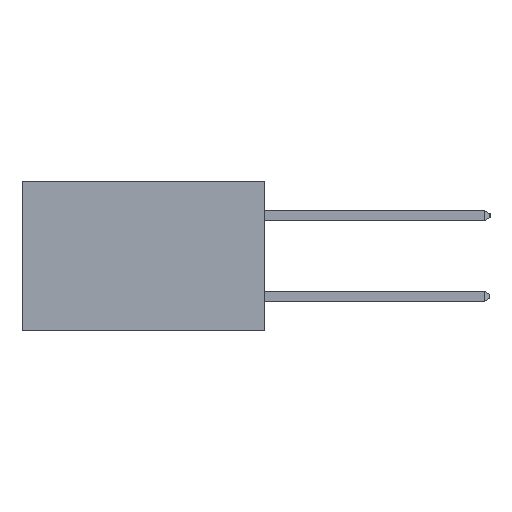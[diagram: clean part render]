
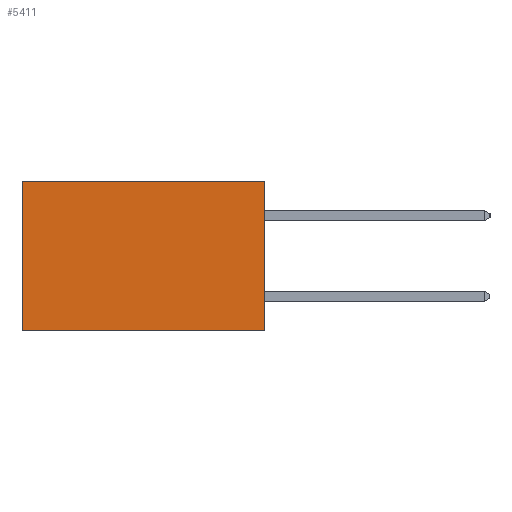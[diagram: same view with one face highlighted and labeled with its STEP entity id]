
A CAD part, left-side view. The second image highlights one B-rep face of the part: STEP entity #5411.
In plain terms, the highlighted planar face has unit normal (-1, 0, 0).
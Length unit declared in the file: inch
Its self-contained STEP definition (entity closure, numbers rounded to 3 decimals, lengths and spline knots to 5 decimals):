
#202 = VECTOR ( 'NONE', #15864, 39.37008 ) ;
#909 = EDGE_CURVE ( 'NONE', #8495, #8430, #10309, .T. ) ;
#1113 = DIRECTION ( 'NONE',  ( 1., 0., 0. ) ) ;
#1303 = CARTESIAN_POINT ( 'NONE',  ( 0.2615, 0., -0.37 ) ) ;
#1357 = LINE ( 'NONE', #3904, #6121 ) ;
#1825 = LINE ( 'NONE', #8540, #7843 ) ;
#2443 = DIRECTION ( 'NONE',  ( 0., 0., -1. ) ) ;
#2485 = ORIENTED_EDGE ( 'NONE', *, *, #9962, .T. ) ;
#3887 = AXIS2_PLACEMENT_3D ( 'NONE', #6572, #1113, #17454 ) ;
#3904 = CARTESIAN_POINT ( 'NONE',  ( 0.2615, 0., 0. ) ) ;
#4393 = EDGE_CURVE ( 'NONE', #8430, #11724, #10046, .T. ) ;
#4702 = ORIENTED_EDGE ( 'NONE', *, *, #5030, .T. ) ;
#5030 = EDGE_CURVE ( 'NONE', #6061, #11724, #1825, .T. ) ;
#5411 = ADVANCED_FACE ( 'NONE', ( #8099 ), #13270, .F. ) ;
#6061 = VERTEX_POINT ( 'NONE', #8173 ) ;
#6121 = VECTOR ( 'NONE', #13860, 39.37008 ) ;
#6231 = CARTESIAN_POINT ( 'NONE',  ( 0.2615, 0., -0.37 ) ) ;
#6572 = CARTESIAN_POINT ( 'NONE',  ( 0.2615, 0., -0.37 ) ) ;
#6700 = VECTOR ( 'NONE', #2443, 39.37008 ) ;
#7843 = VECTOR ( 'NONE', #12641, 39.37008 ) ;
#8099 = FACE_OUTER_BOUND ( 'NONE', #14757, .T. ) ;
#8173 = CARTESIAN_POINT ( 'NONE',  ( 0.2615, 0.6, 0. ) ) ;
#8430 = VERTEX_POINT ( 'NONE', #1303 ) ;
#8495 = VERTEX_POINT ( 'NONE', #13818 ) ;
#8540 = CARTESIAN_POINT ( 'NONE',  ( 0.2615, 0.6, -0.37 ) ) ;
#9392 = ORIENTED_EDGE ( 'NONE', *, *, #909, .F. ) ;
#9962 = EDGE_CURVE ( 'NONE', #8495, #6061, #1357, .T. ) ;
#10046 = LINE ( 'NONE', #6231, #202 ) ;
#10309 = LINE ( 'NONE', #15767, #6700 ) ;
#10592 = CARTESIAN_POINT ( 'NONE',  ( 0.2615, 0.6, -0.37 ) ) ;
#11724 = VERTEX_POINT ( 'NONE', #10592 ) ;
#12641 = DIRECTION ( 'NONE',  ( 0., 0., -1. ) ) ;
#13270 = PLANE ( 'NONE',  #3887 ) ;
#13818 = CARTESIAN_POINT ( 'NONE',  ( 0.2615, 0., 0. ) ) ;
#13860 = DIRECTION ( 'NONE',  ( 0., 1., 0. ) ) ;
#14757 = EDGE_LOOP ( 'NONE', ( #4702, #15365, #9392, #2485 ) ) ;
#15365 = ORIENTED_EDGE ( 'NONE', *, *, #4393, .F. ) ;
#15767 = CARTESIAN_POINT ( 'NONE',  ( 0.2615, 0., -0.37 ) ) ;
#15864 = DIRECTION ( 'NONE',  ( 0., 1., 0. ) ) ;
#17454 = DIRECTION ( 'NONE',  ( 0., 0., -1. ) ) ;
